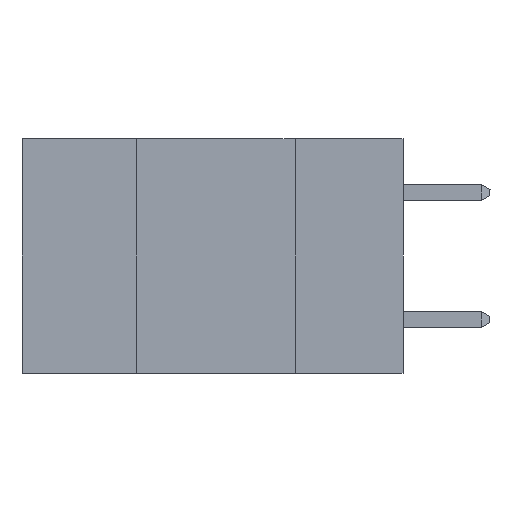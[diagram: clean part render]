
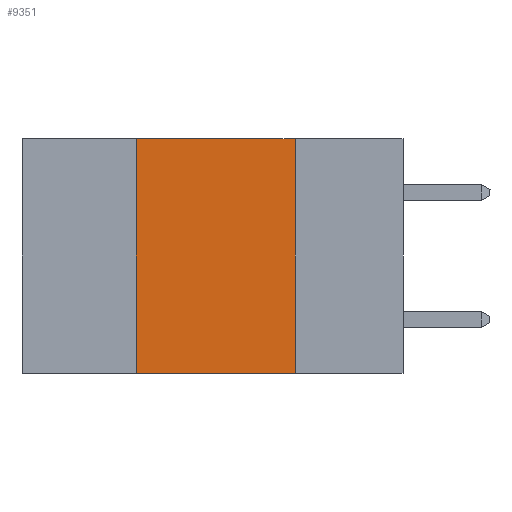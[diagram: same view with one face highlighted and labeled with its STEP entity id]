
A CAD part, left-side view. The second image highlights one B-rep face of the part: STEP entity #9351.
In plain terms, the highlighted planar face has unit normal (-1, 0, 0).
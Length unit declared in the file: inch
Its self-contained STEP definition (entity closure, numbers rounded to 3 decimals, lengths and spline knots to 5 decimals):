
#164 = ORIENTED_EDGE ( 'NONE', *, *, #22773, .F. ) ;
#421 = CARTESIAN_POINT ( 'NONE',  ( 0., 0.6, -0.37 ) ) ;
#664 = LINE ( 'NONE', #19103, #23117 ) ;
#1174 = LINE ( 'NONE', #8660, #17845 ) ;
#1946 = DIRECTION ( 'NONE',  ( 0., 0., -1. ) ) ;
#3874 = EDGE_CURVE ( 'NONE', #10348, #13892, #20183, .T. ) ;
#4184 = DIRECTION ( 'NONE',  ( 0., 0., -1. ) ) ;
#4751 = CARTESIAN_POINT ( 'NONE',  ( 0., 0.42, 0. ) ) ;
#4897 = VECTOR ( 'NONE', #19912, 39.37008 ) ;
#8007 = AXIS2_PLACEMENT_3D ( 'NONE', #27960, #14986, #1946 ) ;
#8620 = DIRECTION ( 'NONE',  ( 0., 0., 1. ) ) ;
#8660 = CARTESIAN_POINT ( 'NONE',  ( 0., 0.6, 0. ) ) ;
#9161 = ORIENTED_EDGE ( 'NONE', *, *, #3874, .F. ) ;
#9351 = ADVANCED_FACE ( 'NONE', ( #24534 ), #25813, .F. ) ;
#10348 = VERTEX_POINT ( 'NONE', #22475 ) ;
#10663 = CARTESIAN_POINT ( 'NONE',  ( 0., 0.42, -0.37 ) ) ;
#12802 = EDGE_CURVE ( 'NONE', #25482, #13892, #15117, .T. ) ;
#13892 = VERTEX_POINT ( 'NONE', #16386 ) ;
#14986 = DIRECTION ( 'NONE',  ( 1., 0., 0. ) ) ;
#15117 = LINE ( 'NONE', #421, #4897 ) ;
#15670 = VERTEX_POINT ( 'NONE', #4751 ) ;
#16386 = CARTESIAN_POINT ( 'NONE',  ( 0., 0.17, -0.37 ) ) ;
#17845 = VECTOR ( 'NONE', #25898, 39.37008 ) ;
#19103 = CARTESIAN_POINT ( 'NONE',  ( 0., 0.42, 0. ) ) ;
#19912 = DIRECTION ( 'NONE',  ( 0., -1., 0. ) ) ;
#20151 = ORIENTED_EDGE ( 'NONE', *, *, #25435, .F. ) ;
#20183 = LINE ( 'NONE', #21347, #23260 ) ;
#21347 = CARTESIAN_POINT ( 'NONE',  ( 0., 0.17, 0. ) ) ;
#22475 = CARTESIAN_POINT ( 'NONE',  ( 0., 0.17, 0. ) ) ;
#22773 = EDGE_CURVE ( 'NONE', #25482, #15670, #664, .T. ) ;
#23117 = VECTOR ( 'NONE', #8620, 39.37008 ) ;
#23248 = EDGE_LOOP ( 'NONE', ( #9161, #20151, #164, #24160 ) ) ;
#23260 = VECTOR ( 'NONE', #4184, 39.37008 ) ;
#24160 = ORIENTED_EDGE ( 'NONE', *, *, #12802, .T. ) ;
#24534 = FACE_OUTER_BOUND ( 'NONE', #23248, .T. ) ;
#25435 = EDGE_CURVE ( 'NONE', #15670, #10348, #1174, .T. ) ;
#25482 = VERTEX_POINT ( 'NONE', #10663 ) ;
#25813 = PLANE ( 'NONE',  #8007 ) ;
#25898 = DIRECTION ( 'NONE',  ( 0., -1., 0. ) ) ;
#27960 = CARTESIAN_POINT ( 'NONE',  ( 0., 0.6, 0. ) ) ;
